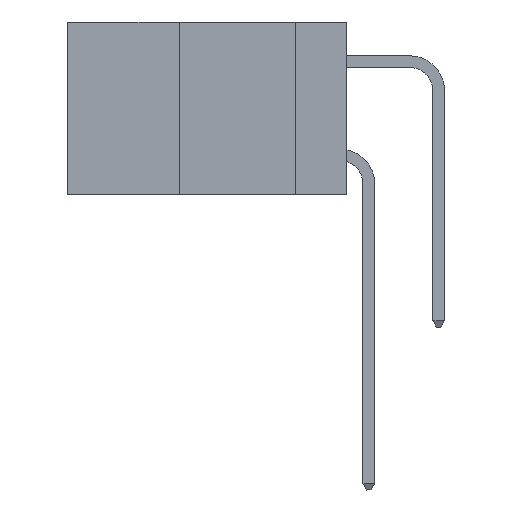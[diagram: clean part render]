
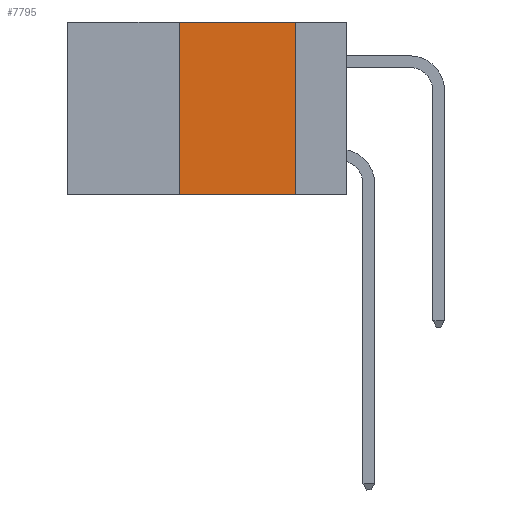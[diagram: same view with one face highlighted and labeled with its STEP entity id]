
A CAD part, left-side view. The second image highlights one B-rep face of the part: STEP entity #7795.
In plain terms, the highlighted planar face has unit normal (-1, 0, 0).
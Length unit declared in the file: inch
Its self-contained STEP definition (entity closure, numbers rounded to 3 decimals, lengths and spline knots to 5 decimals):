
#557 = VECTOR ( 'NONE', #12984, 39.37008 ) ;
#882 = VERTEX_POINT ( 'NONE', #3251 ) ;
#932 = ORIENTED_EDGE ( 'NONE', *, *, #14705, .F. ) ;
#982 = ORIENTED_EDGE ( 'NONE', *, *, #24932, .F. ) ;
#1332 = LINE ( 'NONE', #18245, #6111 ) ;
#2351 = EDGE_LOOP ( 'NONE', ( #932, #982, #19077, #19222 ) ) ;
#3251 = CARTESIAN_POINT ( 'NONE',  ( 0., 0.11, 0. ) ) ;
#5656 = DIRECTION ( 'NONE',  ( 0., 0., 1. ) ) ;
#6111 = VECTOR ( 'NONE', #20173, 39.37008 ) ;
#6806 = CARTESIAN_POINT ( 'NONE',  ( 0., 0.36, -0.37 ) ) ;
#7795 = ADVANCED_FACE ( 'NONE', ( #11136 ), #11936, .F. ) ;
#9557 = VERTEX_POINT ( 'NONE', #6806 ) ;
#9840 = CARTESIAN_POINT ( 'NONE',  ( 0., 0.6, 0. ) ) ;
#10899 = VECTOR ( 'NONE', #5656, 39.37008 ) ;
#11136 = FACE_OUTER_BOUND ( 'NONE', #2351, .T. ) ;
#11575 = EDGE_CURVE ( 'NONE', #9557, #20734, #21614, .T. ) ;
#11868 = CARTESIAN_POINT ( 'NONE',  ( 0., 0.11, 0. ) ) ;
#11936 = PLANE ( 'NONE',  #25037 ) ;
#12984 = DIRECTION ( 'NONE',  ( 0., -1., 0. ) ) ;
#13546 = CARTESIAN_POINT ( 'NONE',  ( 0., 0.36, 0. ) ) ;
#13896 = VECTOR ( 'NONE', #23427, 39.37008 ) ;
#13945 = DIRECTION ( 'NONE',  ( 0., 0., -1. ) ) ;
#14476 = VERTEX_POINT ( 'NONE', #19075 ) ;
#14705 = EDGE_CURVE ( 'NONE', #882, #20734, #19644, .T. ) ;
#16556 = CARTESIAN_POINT ( 'NONE',  ( 0., 0.11, -0.37 ) ) ;
#18245 = CARTESIAN_POINT ( 'NONE',  ( 0., 0.6, 0. ) ) ;
#18867 = CARTESIAN_POINT ( 'NONE',  ( 0., 0.6, -0.37 ) ) ;
#19075 = CARTESIAN_POINT ( 'NONE',  ( 0., 0.36, 0. ) ) ;
#19077 = ORIENTED_EDGE ( 'NONE', *, *, #22110, .F. ) ;
#19222 = ORIENTED_EDGE ( 'NONE', *, *, #11575, .T. ) ;
#19644 = LINE ( 'NONE', #11868, #13896 ) ;
#20173 = DIRECTION ( 'NONE',  ( 0., -1., 0. ) ) ;
#20734 = VERTEX_POINT ( 'NONE', #16556 ) ;
#21614 = LINE ( 'NONE', #18867, #557 ) ;
#22110 = EDGE_CURVE ( 'NONE', #9557, #14476, #23035, .T. ) ;
#23035 = LINE ( 'NONE', #13546, #10899 ) ;
#23427 = DIRECTION ( 'NONE',  ( 0., 0., -1. ) ) ;
#24932 = EDGE_CURVE ( 'NONE', #14476, #882, #1332, .T. ) ;
#25037 = AXIS2_PLACEMENT_3D ( 'NONE', #9840, #25341, #13945 ) ;
#25341 = DIRECTION ( 'NONE',  ( 1., 0., 0. ) ) ;
